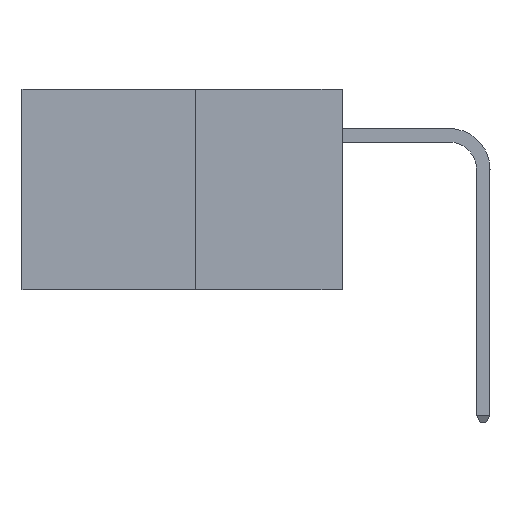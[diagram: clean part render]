
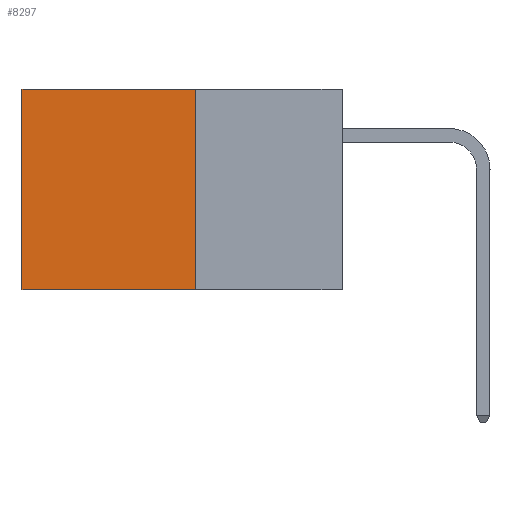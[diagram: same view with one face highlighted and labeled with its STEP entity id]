
A CAD part, left-side view. The second image highlights one B-rep face of the part: STEP entity #8297.
In plain terms, the highlighted planar face has unit normal (-1, 0, 0).
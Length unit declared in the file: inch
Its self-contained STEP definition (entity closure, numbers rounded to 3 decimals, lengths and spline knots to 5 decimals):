
#1117 = CARTESIAN_POINT ( 'NONE',  ( 0.277, 0.27, 0. ) ) ;
#1636 = PLANE ( 'NONE',  #1772 ) ;
#1772 = AXIS2_PLACEMENT_3D ( 'NONE', #2068, #8613, #7201 ) ;
#2068 = CARTESIAN_POINT ( 'NONE',  ( 0.277, 0.27, -0.37 ) ) ;
#2259 = DIRECTION ( 'NONE',  ( 0., 0., -1. ) ) ;
#2270 = VECTOR ( 'NONE', #14491, 39.37008 ) ;
#2271 = EDGE_CURVE ( 'NONE', #13959, #12467, #6728, .T. ) ;
#3727 = ORIENTED_EDGE ( 'NONE', *, *, #10522, .T. ) ;
#4034 = VECTOR ( 'NONE', #11337, 39.37008 ) ;
#4193 = CARTESIAN_POINT ( 'NONE',  ( 0.277, 0.59, 0. ) ) ;
#4757 = LINE ( 'NONE', #8738, #4034 ) ;
#4946 = LINE ( 'NONE', #14505, #2270 ) ;
#5735 = CARTESIAN_POINT ( 'NONE',  ( 0.277, 0.27, -0.37 ) ) ;
#6490 = FACE_OUTER_BOUND ( 'NONE', #12240, .T. ) ;
#6728 = LINE ( 'NONE', #7400, #9670 ) ;
#6936 = LINE ( 'NONE', #9065, #12554 ) ;
#7201 = DIRECTION ( 'NONE',  ( 0., 0., -1. ) ) ;
#7226 = DIRECTION ( 'NONE',  ( 0., 1., 0. ) ) ;
#7342 = EDGE_CURVE ( 'NONE', #13959, #9348, #4946, .T. ) ;
#7400 = CARTESIAN_POINT ( 'NONE',  ( 0.277, 0.27, 0. ) ) ;
#7596 = EDGE_CURVE ( 'NONE', #9348, #14154, #4757, .T. ) ;
#8297 = ADVANCED_FACE ( 'NONE', ( #6490 ), #1636, .F. ) ;
#8329 = ORIENTED_EDGE ( 'NONE', *, *, #2271, .T. ) ;
#8477 = CARTESIAN_POINT ( 'NONE',  ( 0.277, 0.59, -0.37 ) ) ;
#8613 = DIRECTION ( 'NONE',  ( 1., 0., 0. ) ) ;
#8738 = CARTESIAN_POINT ( 'NONE',  ( 0.277, 0.27, -0.37 ) ) ;
#9065 = CARTESIAN_POINT ( 'NONE',  ( 0.277, 0.59, -0.37 ) ) ;
#9348 = VERTEX_POINT ( 'NONE', #5735 ) ;
#9670 = VECTOR ( 'NONE', #7226, 39.37008 ) ;
#10522 = EDGE_CURVE ( 'NONE', #12467, #14154, #6936, .T. ) ;
#11112 = ORIENTED_EDGE ( 'NONE', *, *, #7342, .F. ) ;
#11337 = DIRECTION ( 'NONE',  ( 0., 1., 0. ) ) ;
#12240 = EDGE_LOOP ( 'NONE', ( #3727, #12449, #11112, #8329 ) ) ;
#12449 = ORIENTED_EDGE ( 'NONE', *, *, #7596, .F. ) ;
#12467 = VERTEX_POINT ( 'NONE', #4193 ) ;
#12554 = VECTOR ( 'NONE', #2259, 39.37008 ) ;
#13959 = VERTEX_POINT ( 'NONE', #1117 ) ;
#14154 = VERTEX_POINT ( 'NONE', #8477 ) ;
#14491 = DIRECTION ( 'NONE',  ( 0., 0., -1. ) ) ;
#14505 = CARTESIAN_POINT ( 'NONE',  ( 0.277, 0.27, -0.37 ) ) ;
